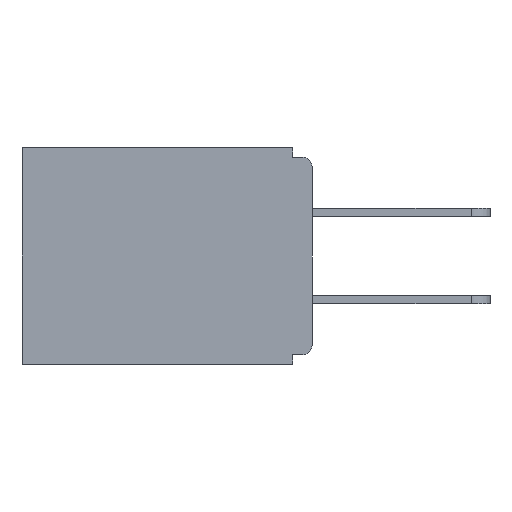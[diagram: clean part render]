
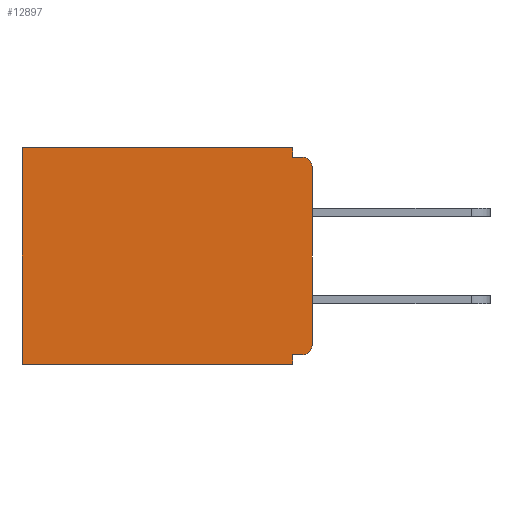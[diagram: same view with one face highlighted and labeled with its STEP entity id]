
A CAD part, left-side view. The second image highlights one B-rep face of the part: STEP entity #12897.
In plain terms, the highlighted planar face has unit normal (-1, 0, 0).
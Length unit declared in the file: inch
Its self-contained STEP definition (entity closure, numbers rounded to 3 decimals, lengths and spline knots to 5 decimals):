
#253 = CARTESIAN_POINT ( 'NONE',  ( 0.298, 0.031, -0.328 ) ) ;
#312 = EDGE_CURVE ( 'NONE', #2422, #464, #14762, .T. ) ;
#464 = VERTEX_POINT ( 'NONE', #12983 ) ;
#825 = ORIENTED_EDGE ( 'NONE', *, *, #2507, .F. ) ;
#1042 = CARTESIAN_POINT ( 'NONE',  ( 0.298, 0., -0.015 ) ) ;
#1256 = EDGE_LOOP ( 'NONE', ( #1480, #8524, #14479, #12632, #14357, #7859, #825, #15359, #17362, #8339 ) ) ;
#1347 = PLANE ( 'NONE',  #11511 ) ;
#1453 = DIRECTION ( 'NONE',  ( 0., 0., -1. ) ) ;
#1480 = ORIENTED_EDGE ( 'NONE', *, *, #2104, .T. ) ;
#2104 = EDGE_CURVE ( 'NONE', #15439, #9556, #14691, .T. ) ;
#2422 = VERTEX_POINT ( 'NONE', #9244 ) ;
#2430 = CARTESIAN_POINT ( 'NONE',  ( 0.298, 0.46, -0.343 ) ) ;
#2507 = EDGE_CURVE ( 'NONE', #7413, #10204, #13221, .T. ) ;
#2534 = CARTESIAN_POINT ( 'NONE',  ( 0.298, 0.031, 0. ) ) ;
#2659 = LINE ( 'NONE', #4871, #12886 ) ;
#2734 = VECTOR ( 'NONE', #8660, 39.37008 ) ;
#3119 = VECTOR ( 'NONE', #15759, 39.37008 ) ;
#3342 = EDGE_CURVE ( 'NONE', #10204, #12284, #10465, .T. ) ;
#3560 = VERTEX_POINT ( 'NONE', #11899 ) ;
#3566 = EDGE_CURVE ( 'NONE', #16194, #9556, #10248, .T. ) ;
#4010 = DIRECTION ( 'NONE',  ( 0., 0., -1. ) ) ;
#4089 = DIRECTION ( 'NONE',  ( 0., 1., 0. ) ) ;
#4110 = VECTOR ( 'NONE', #4089, 39.37008 ) ;
#4419 = VECTOR ( 'NONE', #9193, 39.37008 ) ;
#4599 = DIRECTION ( 'NONE',  ( 0., 0., -1. ) ) ;
#4771 = DIRECTION ( 'NONE',  ( -1., 0., 0. ) ) ;
#4871 = CARTESIAN_POINT ( 'NONE',  ( 0.298, 0., 0. ) ) ;
#5592 = VERTEX_POINT ( 'NONE', #2534 ) ;
#5882 = CARTESIAN_POINT ( 'NONE',  ( 0.298, 0.015, -0.03 ) ) ;
#6052 = EDGE_CURVE ( 'NONE', #2422, #7413, #10205, .T. ) ;
#6454 = CARTESIAN_POINT ( 'NONE',  ( 0.298, 0., -0.328 ) ) ;
#6535 = EDGE_CURVE ( 'NONE', #5592, #16194, #10991, .T. ) ;
#6577 = CARTESIAN_POINT ( 'NONE',  ( 0.298, 0.031, -0.343 ) ) ;
#6674 = CARTESIAN_POINT ( 'NONE',  ( 0.298, 0.015, -0.015 ) ) ;
#7197 = AXIS2_PLACEMENT_3D ( 'NONE', #16700, #10484, #12762 ) ;
#7413 = VERTEX_POINT ( 'NONE', #253 ) ;
#7595 = CARTESIAN_POINT ( 'NONE',  ( 0.298, 0., -0.03 ) ) ;
#7859 = ORIENTED_EDGE ( 'NONE', *, *, #3342, .F. ) ;
#8339 = ORIENTED_EDGE ( 'NONE', *, *, #11191, .F. ) ;
#8415 = VECTOR ( 'NONE', #1453, 39.37008 ) ;
#8524 = ORIENTED_EDGE ( 'NONE', *, *, #3566, .F. ) ;
#8660 = DIRECTION ( 'NONE',  ( 0., 0., -1. ) ) ;
#9193 = DIRECTION ( 'NONE',  ( 0., -1., 0. ) ) ;
#9244 = CARTESIAN_POINT ( 'NONE',  ( 0.298, 0.015, -0.328 ) ) ;
#9314 = CARTESIAN_POINT ( 'NONE',  ( 0.298, 0., 0. ) ) ;
#9556 = VERTEX_POINT ( 'NONE', #6674 ) ;
#9628 = CARTESIAN_POINT ( 'NONE',  ( 0.298, 0., 0. ) ) ;
#9941 = DIRECTION ( 'NONE',  ( 0., 1., 0. ) ) ;
#10143 = DIRECTION ( 'NONE',  ( 0., 0., -1. ) ) ;
#10204 = VERTEX_POINT ( 'NONE', #6577 ) ;
#10205 = LINE ( 'NONE', #6454, #3119 ) ;
#10248 = LINE ( 'NONE', #1042, #4419 ) ;
#10351 = LINE ( 'NONE', #9628, #4110 ) ;
#10465 = LINE ( 'NONE', #15189, #12118 ) ;
#10484 = DIRECTION ( 'NONE',  ( -1., 0., 0. ) ) ;
#10991 = LINE ( 'NONE', #16620, #14984 ) ;
#11191 = EDGE_CURVE ( 'NONE', #15439, #464, #2659, .T. ) ;
#11511 = AXIS2_PLACEMENT_3D ( 'NONE', #9314, #11853, #4010 ) ;
#11824 = EDGE_CURVE ( 'NONE', #5592, #3560, #10351, .T. ) ;
#11853 = DIRECTION ( 'NONE',  ( 1., 0., 0. ) ) ;
#11899 = CARTESIAN_POINT ( 'NONE',  ( 0.298, 0.46, 0. ) ) ;
#12118 = VECTOR ( 'NONE', #9941, 39.37008 ) ;
#12176 = CARTESIAN_POINT ( 'NONE',  ( 0.298, 0.031, -0.343 ) ) ;
#12284 = VERTEX_POINT ( 'NONE', #2430 ) ;
#12526 = LINE ( 'NONE', #16604, #2734 ) ;
#12632 = ORIENTED_EDGE ( 'NONE', *, *, #11824, .T. ) ;
#12762 = DIRECTION ( 'NONE',  ( 0., 0., -1. ) ) ;
#12886 = VECTOR ( 'NONE', #10143, 39.37008 ) ;
#12897 = ADVANCED_FACE ( 'NONE', ( #15778 ), #1347, .F. ) ;
#12983 = CARTESIAN_POINT ( 'NONE',  ( 0.298, 0., -0.313 ) ) ;
#13221 = LINE ( 'NONE', #12176, #8415 ) ;
#14357 = ORIENTED_EDGE ( 'NONE', *, *, #15250, .T. ) ;
#14479 = ORIENTED_EDGE ( 'NONE', *, *, #6535, .F. ) ;
#14691 = CIRCLE ( 'NONE', #17098, 0.015 ) ;
#14712 = CARTESIAN_POINT ( 'NONE',  ( 0.298, 0.031, -0.015 ) ) ;
#14762 = CIRCLE ( 'NONE', #7197, 0.015 ) ;
#14984 = VECTOR ( 'NONE', #4599, 39.37008 ) ;
#15189 = CARTESIAN_POINT ( 'NONE',  ( 0.298, 0., -0.343 ) ) ;
#15250 = EDGE_CURVE ( 'NONE', #3560, #12284, #12526, .T. ) ;
#15292 = DIRECTION ( 'NONE',  ( 0., 0., -1. ) ) ;
#15359 = ORIENTED_EDGE ( 'NONE', *, *, #6052, .F. ) ;
#15439 = VERTEX_POINT ( 'NONE', #7595 ) ;
#15759 = DIRECTION ( 'NONE',  ( 0., 1., 0. ) ) ;
#15778 = FACE_OUTER_BOUND ( 'NONE', #1256, .T. ) ;
#16194 = VERTEX_POINT ( 'NONE', #14712 ) ;
#16604 = CARTESIAN_POINT ( 'NONE',  ( 0.298, 0.46, 0. ) ) ;
#16620 = CARTESIAN_POINT ( 'NONE',  ( 0.298, 0.031, -0.343 ) ) ;
#16700 = CARTESIAN_POINT ( 'NONE',  ( 0.298, 0.015, -0.313 ) ) ;
#17098 = AXIS2_PLACEMENT_3D ( 'NONE', #5882, #4771, #15292 ) ;
#17362 = ORIENTED_EDGE ( 'NONE', *, *, #312, .T. ) ;
